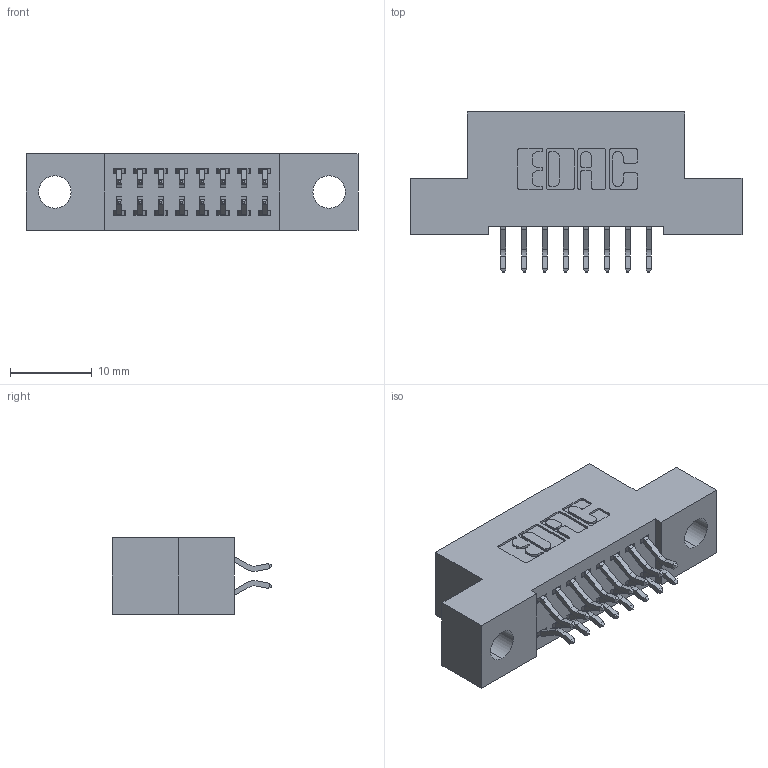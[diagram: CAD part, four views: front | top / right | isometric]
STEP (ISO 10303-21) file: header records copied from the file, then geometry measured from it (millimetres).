
FILE_DESCRIPTION (( 'STEP AP203' ), '1' );
FILE_NAME ('392-016-556-204.STEP', '2019-10-07T03:23:43', ( '' ), ( '' ), 'SwSTEP 2.0', 'SolidWorks 2016', '' );
FILE_SCHEMA (( 'CONFIG_CONTROL_DESIGN' ));
Length unit declared in the file: inch
Products named in the file (3): 392-016-556-204; 342 Part_.156 TH; 345-292-001_556 Tail
Assembly tree (17 placements, depth 2):
  392-016-556-204
    342 Part_.156 TH
    345-292-001_556 Tail  x16
Bounding box: 40.64 x 19.58 x 9.4 mm (x, y, z)
Volume: 3403.1 mm3; surface area: 4510.3 mm2
Topology: 17 solids, 17 shells, 1038 faces, 3067 edges, 2022 vertices
Faces by surface type: plane 706, cylinder 332
Entity records: 9635 total; most frequent: CARTESIAN_POINT 1650, ORIENTED_EDGE 1574, DIRECTION 1459, EDGE_CURVE 787, VECTOR 651, LINE 651, VERTEX_POINT 522, AXIS2_PLACEMENT_3D 404
